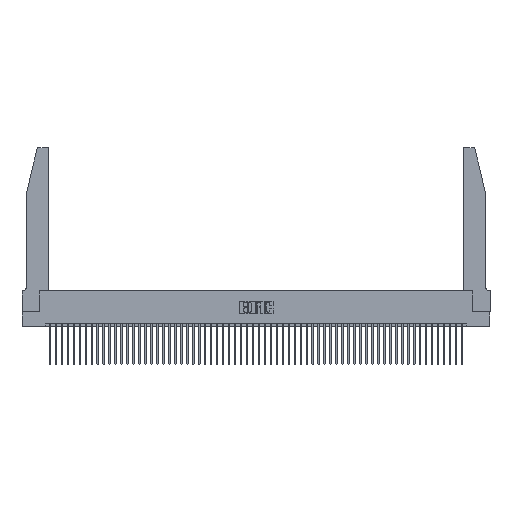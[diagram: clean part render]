
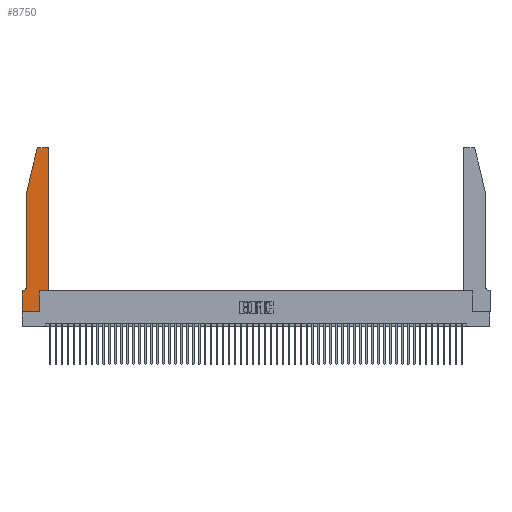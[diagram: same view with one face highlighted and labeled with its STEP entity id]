
A CAD part, top view. The second image highlights one B-rep face of the part: STEP entity #8750.
In plain terms, the highlighted planar face has unit normal (0, 0, 1).
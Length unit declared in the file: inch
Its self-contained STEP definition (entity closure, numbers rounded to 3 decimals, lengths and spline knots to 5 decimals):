
#41 = LINE ( 'NONE', #52891, #9525 ) ;
#332 = DIRECTION ( 'NONE',  ( 0., 1., 0. ) ) ;
#538 = VERTEX_POINT ( 'NONE', #51190 ) ;
#655 = DIRECTION ( 'NONE',  ( 0., 0., -1. ) ) ;
#1018 = CARTESIAN_POINT ( 'NONE',  ( 0.284, 2.75, 0.37 ) ) ;
#2945 = DIRECTION ( 'NONE',  ( 1., 0., 0. ) ) ;
#3473 = CARTESIAN_POINT ( 'NONE',  ( 0.4505, 2.72, 0.37 ) ) ;
#3786 = FACE_OUTER_BOUND ( 'NONE', #37676, .T. ) ;
#4257 = AXIS2_PLACEMENT_3D ( 'NONE', #33682, #38225, #16670 ) ;
#4766 = CARTESIAN_POINT ( 'NONE',  ( 0., 0., 0.37 ) ) ;
#4824 = VERTEX_POINT ( 'NONE', #32808 ) ;
#5149 = DIRECTION ( 'NONE',  ( 0., 1., 0. ) ) ;
#6440 = DIRECTION ( 'NONE',  ( 1., 0., 0. ) ) ;
#6602 = LINE ( 'NONE', #41021, #32296 ) ;
#8030 = LINE ( 'NONE', #10018, #43161 ) ;
#8603 = DIRECTION ( 'NONE',  ( -1., 0., 0. ) ) ;
#8750 = ADVANCED_FACE ( 'NONE', ( #3786 ), #20118, .T. ) ;
#8761 = CARTESIAN_POINT ( 'NONE',  ( 0.0055, 0.42, 0.37 ) ) ;
#9525 = VECTOR ( 'NONE', #5149, 39.37008 ) ;
#9734 = VERTEX_POINT ( 'NONE', #1018 ) ;
#10018 = CARTESIAN_POINT ( 'NONE',  ( 0.0755, 2., 0.37 ) ) ;
#11287 = EDGE_CURVE ( 'NONE', #14555, #34835, #18984, .T. ) ;
#11420 = DIRECTION ( 'NONE',  ( 0., 0., 1. ) ) ;
#11431 = CARTESIAN_POINT ( 'NONE',  ( 0.0755, 0.42, 0.37 ) ) ;
#11618 = CARTESIAN_POINT ( 'NONE',  ( 0., 0.35, 0.37 ) ) ;
#12511 = VERTEX_POINT ( 'NONE', #34634 ) ;
#12918 = DIRECTION ( 'NONE',  ( -1., 0., 0. ) ) ;
#13225 = VERTEX_POINT ( 'NONE', #3473 ) ;
#13796 = EDGE_CURVE ( 'NONE', #34835, #38357, #27363, .T. ) ;
#14555 = VERTEX_POINT ( 'NONE', #11431 ) ;
#14932 = DIRECTION ( 'NONE',  ( -1., 0., 0. ) ) ;
#14971 = VERTEX_POINT ( 'NONE', #39762 ) ;
#15565 = EDGE_CURVE ( 'NONE', #38357, #48809, #46086, .T. ) ;
#16670 = DIRECTION ( 'NONE',  ( 1., 0., 0. ) ) ;
#18080 = EDGE_CURVE ( 'NONE', #12511, #32020, #45179, .T. ) ;
#18984 = CIRCLE ( 'NONE', #32528, 0.07 ) ;
#19728 = EDGE_CURVE ( 'NONE', #32020, #13225, #41, .T. ) ;
#19772 = ORIENTED_EDGE ( 'NONE', *, *, #11287, .T. ) ;
#19814 = DIRECTION ( 'NONE',  ( 0., 0., 1. ) ) ;
#19957 = AXIS2_PLACEMENT_3D ( 'NONE', #45721, #19814, #50586 ) ;
#20118 = PLANE ( 'NONE',  #21717 ) ;
#20640 = VECTOR ( 'NONE', #8603, 39.37008 ) ;
#21673 = DIRECTION ( 'NONE',  ( 1., 0., 0. ) ) ;
#21717 = AXIS2_PLACEMENT_3D ( 'NONE', #11618, #11420, #2945 ) ;
#21727 = EDGE_CURVE ( 'NONE', #14971, #538, #8030, .T. ) ;
#22014 = LINE ( 'NONE', #51844, #20640 ) ;
#22810 = CARTESIAN_POINT ( 'NONE',  ( 0.2865, 0., 0.37 ) ) ;
#22840 = VECTOR ( 'NONE', #21673, 39.37008 ) ;
#23091 = VECTOR ( 'NONE', #332, 39.37008 ) ;
#23600 = ORIENTED_EDGE ( 'NONE', *, *, #45084, .T. ) ;
#23727 = DIRECTION ( 'NONE',  ( 0., -1., 0. ) ) ;
#24725 = ORIENTED_EDGE ( 'NONE', *, *, #15565, .T. ) ;
#25676 = EDGE_CURVE ( 'NONE', #9734, #14971, #48000, .T. ) ;
#27154 = VECTOR ( 'NONE', #23727, 39.37008 ) ;
#27363 = LINE ( 'NONE', #53654, #55727 ) ;
#29322 = ORIENTED_EDGE ( 'NONE', *, *, #39117, .T. ) ;
#31084 = EDGE_CURVE ( 'NONE', #55850, #12511, #33228, .T. ) ;
#31924 = CARTESIAN_POINT ( 'NONE',  ( 0., 0., 0.37 ) ) ;
#32020 = VERTEX_POINT ( 'NONE', #51958 ) ;
#32296 = VECTOR ( 'NONE', #6440, 39.37008 ) ;
#32528 = AXIS2_PLACEMENT_3D ( 'NONE', #8761, #655, #12918 ) ;
#32808 = CARTESIAN_POINT ( 'NONE',  ( 0.4205, 2.75, 0.37 ) ) ;
#33228 = LINE ( 'NONE', #43412, #23091 ) ;
#33362 = DIRECTION ( 'NONE',  ( -0.239, -0.971, 0. ) ) ;
#33682 = CARTESIAN_POINT ( 'NONE',  ( 0.4205, 2.72, 0.37 ) ) ;
#34634 = CARTESIAN_POINT ( 'NONE',  ( 0.2865, 0.35, 0.37 ) ) ;
#34835 = VERTEX_POINT ( 'NONE', #38430 ) ;
#34904 = CARTESIAN_POINT ( 'NONE',  ( 0.4505, 0.35, 0.37 ) ) ;
#37676 = EDGE_LOOP ( 'NONE', ( #49800, #54372, #39458, #54483, #19772, #50133, #24725, #29322, #46451, #54310, #52763, #23600 ) ) ;
#38225 = DIRECTION ( 'NONE',  ( 0., 0., 1. ) ) ;
#38357 = VERTEX_POINT ( 'NONE', #43181 ) ;
#38430 = CARTESIAN_POINT ( 'NONE',  ( 0.0055, 0.35, 0.37 ) ) ;
#39117 = EDGE_CURVE ( 'NONE', #48809, #55850, #6602, .T. ) ;
#39458 = ORIENTED_EDGE ( 'NONE', *, *, #21727, .T. ) ;
#39762 = CARTESIAN_POINT ( 'NONE',  ( 0.25487, 2.72718, 0.37 ) ) ;
#40210 = EDGE_CURVE ( 'NONE', #4824, #9734, #22014, .T. ) ;
#41021 = CARTESIAN_POINT ( 'NONE',  ( 0., 0., 0.37 ) ) ;
#43161 = VECTOR ( 'NONE', #33362, 39.37008 ) ;
#43181 = CARTESIAN_POINT ( 'NONE',  ( 0., 0.35, 0.37 ) ) ;
#43412 = CARTESIAN_POINT ( 'NONE',  ( 0.2865, 0.35, 0.37 ) ) ;
#45084 = EDGE_CURVE ( 'NONE', #13225, #4824, #47203, .T. ) ;
#45179 = LINE ( 'NONE', #34904, #22840 ) ;
#45285 = LINE ( 'NONE', #45454, #46634 ) ;
#45454 = CARTESIAN_POINT ( 'NONE',  ( 0.0755, 2., 0.37 ) ) ;
#45721 = CARTESIAN_POINT ( 'NONE',  ( 0.284, 2.72, 0.37 ) ) ;
#46086 = LINE ( 'NONE', #4766, #27154 ) ;
#46451 = ORIENTED_EDGE ( 'NONE', *, *, #31084, .T. ) ;
#46634 = VECTOR ( 'NONE', #49209, 39.37008 ) ;
#47203 = CIRCLE ( 'NONE', #4257, 0.03 ) ;
#48000 = CIRCLE ( 'NONE', #19957, 0.03 ) ;
#48809 = VERTEX_POINT ( 'NONE', #31924 ) ;
#49209 = DIRECTION ( 'NONE',  ( 0., -1., 0. ) ) ;
#49800 = ORIENTED_EDGE ( 'NONE', *, *, #40210, .T. ) ;
#50133 = ORIENTED_EDGE ( 'NONE', *, *, #13796, .T. ) ;
#50586 = DIRECTION ( 'NONE',  ( 1., 0., 0. ) ) ;
#51190 = CARTESIAN_POINT ( 'NONE',  ( 0.0755, 2., 0.37 ) ) ;
#51844 = CARTESIAN_POINT ( 'NONE',  ( 0.2605, 2.75, 0.37 ) ) ;
#51958 = CARTESIAN_POINT ( 'NONE',  ( 0.4505, 0.35, 0.37 ) ) ;
#52763 = ORIENTED_EDGE ( 'NONE', *, *, #19728, .T. ) ;
#52891 = CARTESIAN_POINT ( 'NONE',  ( 0.4505, 0.35, 0.37 ) ) ;
#53654 = CARTESIAN_POINT ( 'NONE',  ( 0.0755, 0.35, 0.37 ) ) ;
#54072 = EDGE_CURVE ( 'NONE', #538, #14555, #45285, .T. ) ;
#54310 = ORIENTED_EDGE ( 'NONE', *, *, #18080, .T. ) ;
#54372 = ORIENTED_EDGE ( 'NONE', *, *, #25676, .T. ) ;
#54483 = ORIENTED_EDGE ( 'NONE', *, *, #54072, .T. ) ;
#55727 = VECTOR ( 'NONE', #14932, 39.37008 ) ;
#55850 = VERTEX_POINT ( 'NONE', #22810 ) ;
